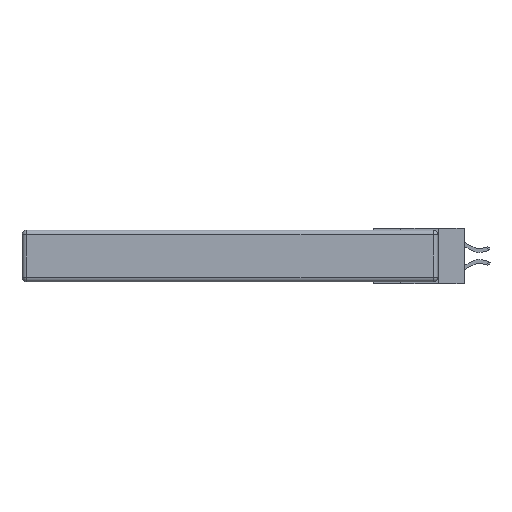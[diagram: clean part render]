
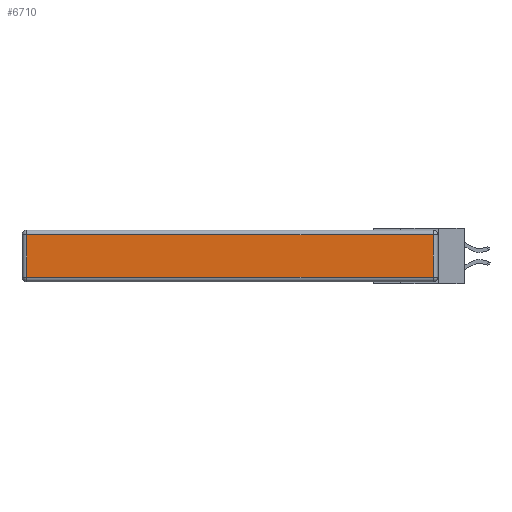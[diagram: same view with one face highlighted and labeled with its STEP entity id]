
A CAD part, left-side view. The second image highlights one B-rep face of the part: STEP entity #6710.
In plain terms, the highlighted planar face has unit normal (-1, 0, 0).
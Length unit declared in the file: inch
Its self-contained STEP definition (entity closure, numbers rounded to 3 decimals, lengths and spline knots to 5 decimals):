
#139 = LINE ( 'NONE', #11825, #8010 ) ;
#1270 = PLANE ( 'NONE',  #10469 ) ;
#1561 = ORIENTED_EDGE ( 'NONE', *, *, #10529, .T. ) ;
#2037 = VECTOR ( 'NONE', #12482, 39.37008 ) ;
#2213 = ORIENTED_EDGE ( 'NONE', *, *, #10090, .T. ) ;
#3302 = CARTESIAN_POINT ( 'NONE',  ( 0., 0.03, -0.343 ) ) ;
#3478 = VERTEX_POINT ( 'NONE', #5545 ) ;
#3700 = DIRECTION ( 'NONE',  ( 0., 0., -1. ) ) ;
#3787 = CARTESIAN_POINT ( 'NONE',  ( 0., 2.72, -0.313 ) ) ;
#5545 = CARTESIAN_POINT ( 'NONE',  ( 0., 0.03, -0.03 ) ) ;
#5587 = ORIENTED_EDGE ( 'NONE', *, *, #9684, .T. ) ;
#5964 = VERTEX_POINT ( 'NONE', #6895 ) ;
#6222 = EDGE_CURVE ( 'NONE', #3478, #12039, #8955, .T. ) ;
#6310 = LINE ( 'NONE', #7795, #8351 ) ;
#6710 = ADVANCED_FACE ( 'NONE', ( #8446 ), #1270, .T. ) ;
#6895 = CARTESIAN_POINT ( 'NONE',  ( 0., 0.03, -0.313 ) ) ;
#7342 = CARTESIAN_POINT ( 'NONE',  ( 0., 2.72, -0.03 ) ) ;
#7795 = CARTESIAN_POINT ( 'NONE',  ( 0., 2.72, -0.343 ) ) ;
#8010 = VECTOR ( 'NONE', #9873, 39.37008 ) ;
#8351 = VECTOR ( 'NONE', #3700, 39.37008 ) ;
#8446 = FACE_OUTER_BOUND ( 'NONE', #12295, .T. ) ;
#8955 = LINE ( 'NONE', #11635, #10523 ) ;
#9271 = CARTESIAN_POINT ( 'NONE',  ( 0., 0., -0.343 ) ) ;
#9684 = EDGE_CURVE ( 'NONE', #12039, #9697, #6310, .T. ) ;
#9697 = VERTEX_POINT ( 'NONE', #3787 ) ;
#9873 = DIRECTION ( 'NONE',  ( 0., -1., 0. ) ) ;
#10090 = EDGE_CURVE ( 'NONE', #9697, #5964, #139, .T. ) ;
#10469 = AXIS2_PLACEMENT_3D ( 'NONE', #9271, #11493, #12329 ) ;
#10523 = VECTOR ( 'NONE', #11676, 39.37008 ) ;
#10529 = EDGE_CURVE ( 'NONE', #5964, #3478, #11846, .T. ) ;
#10919 = ORIENTED_EDGE ( 'NONE', *, *, #6222, .T. ) ;
#11493 = DIRECTION ( 'NONE',  ( -1., 0., 0. ) ) ;
#11635 = CARTESIAN_POINT ( 'NONE',  ( 0., 2.75, -0.03 ) ) ;
#11676 = DIRECTION ( 'NONE',  ( 0., 1., 0. ) ) ;
#11825 = CARTESIAN_POINT ( 'NONE',  ( 0., 0., -0.313 ) ) ;
#11846 = LINE ( 'NONE', #3302, #2037 ) ;
#12039 = VERTEX_POINT ( 'NONE', #7342 ) ;
#12295 = EDGE_LOOP ( 'NONE', ( #2213, #1561, #10919, #5587 ) ) ;
#12329 = DIRECTION ( 'NONE',  ( 0., 0., 1. ) ) ;
#12482 = DIRECTION ( 'NONE',  ( 0., 0., 1. ) ) ;
